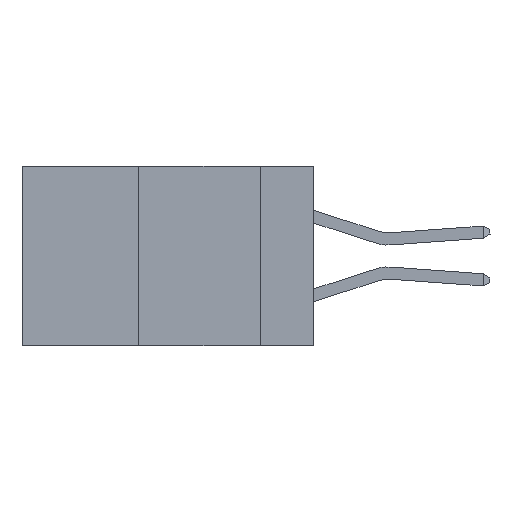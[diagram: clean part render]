
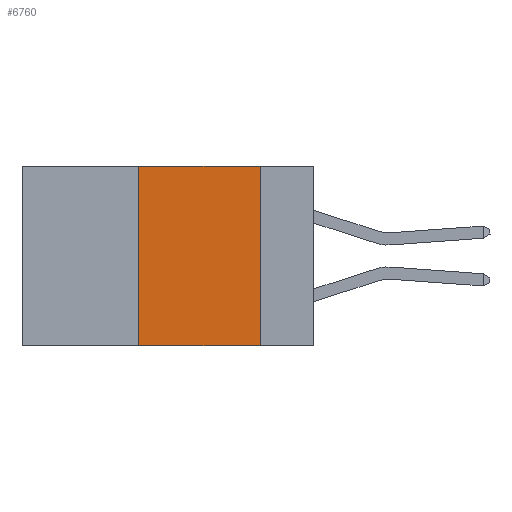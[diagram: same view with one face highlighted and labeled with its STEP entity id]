
A CAD part, left-side view. The second image highlights one B-rep face of the part: STEP entity #6760.
In plain terms, the highlighted planar face has unit normal (-1, 0, 0).
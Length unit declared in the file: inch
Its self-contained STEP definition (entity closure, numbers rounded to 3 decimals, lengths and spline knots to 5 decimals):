
#1212 = EDGE_CURVE ( 'NONE', #1737, #8134, #6768, .T. ) ;
#1675 = VECTOR ( 'NONE', #2789, 39.37008 ) ;
#1737 = VERTEX_POINT ( 'NONE', #9957 ) ;
#2080 = CARTESIAN_POINT ( 'NONE',  ( 0., 0.11, 0. ) ) ;
#2518 = DIRECTION ( 'NONE',  ( 0., 0., -1. ) ) ;
#2750 = DIRECTION ( 'NONE',  ( 0., 0., -1. ) ) ;
#2789 = DIRECTION ( 'NONE',  ( 0., -1., 0. ) ) ;
#2816 = VECTOR ( 'NONE', #2518, 39.37008 ) ;
#3047 = VECTOR ( 'NONE', #8664, 39.37008 ) ;
#3432 = LINE ( 'NONE', #11617, #3047 ) ;
#3678 = ORIENTED_EDGE ( 'NONE', *, *, #9001, .F. ) ;
#3899 = ORIENTED_EDGE ( 'NONE', *, *, #10842, .F. ) ;
#5187 = EDGE_CURVE ( 'NONE', #1737, #9981, #3432, .T. ) ;
#5891 = CARTESIAN_POINT ( 'NONE',  ( 0., 0.36, 0. ) ) ;
#5970 = CARTESIAN_POINT ( 'NONE',  ( 0., 0.6, 0. ) ) ;
#6547 = EDGE_LOOP ( 'NONE', ( #3899, #3678, #6586, #7627 ) ) ;
#6586 = ORIENTED_EDGE ( 'NONE', *, *, #1212, .F. ) ;
#6653 = FACE_OUTER_BOUND ( 'NONE', #6547, .T. ) ;
#6760 = ADVANCED_FACE ( 'NONE', ( #6653 ), #7919, .F. ) ;
#6768 = LINE ( 'NONE', #9015, #12848 ) ;
#7229 = CARTESIAN_POINT ( 'NONE',  ( 0., 0.11, -0.37 ) ) ;
#7627 = ORIENTED_EDGE ( 'NONE', *, *, #5187, .T. ) ;
#7919 = PLANE ( 'NONE',  #8154 ) ;
#8134 = VERTEX_POINT ( 'NONE', #5891 ) ;
#8154 = AXIS2_PLACEMENT_3D ( 'NONE', #12101, #10184, #2750 ) ;
#8664 = DIRECTION ( 'NONE',  ( 0., -1., 0. ) ) ;
#9001 = EDGE_CURVE ( 'NONE', #8134, #9089, #12135, .T. ) ;
#9015 = CARTESIAN_POINT ( 'NONE',  ( 0., 0.36, 0. ) ) ;
#9089 = VERTEX_POINT ( 'NONE', #2080 ) ;
#9814 = CARTESIAN_POINT ( 'NONE',  ( 0., 0.11, 0. ) ) ;
#9847 = DIRECTION ( 'NONE',  ( 0., 0., 1. ) ) ;
#9957 = CARTESIAN_POINT ( 'NONE',  ( 0., 0.36, -0.37 ) ) ;
#9981 = VERTEX_POINT ( 'NONE', #7229 ) ;
#10184 = DIRECTION ( 'NONE',  ( 1., 0., 0. ) ) ;
#10842 = EDGE_CURVE ( 'NONE', #9089, #9981, #12878, .T. ) ;
#11617 = CARTESIAN_POINT ( 'NONE',  ( 0., 0.6, -0.37 ) ) ;
#12101 = CARTESIAN_POINT ( 'NONE',  ( 0., 0.6, 0. ) ) ;
#12135 = LINE ( 'NONE', #5970, #1675 ) ;
#12848 = VECTOR ( 'NONE', #9847, 39.37008 ) ;
#12878 = LINE ( 'NONE', #9814, #2816 ) ;
